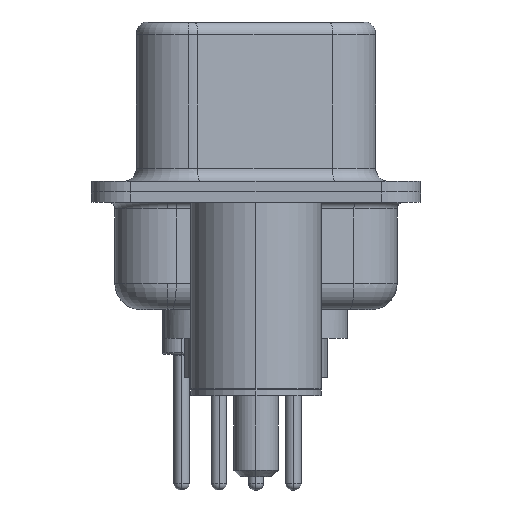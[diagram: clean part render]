
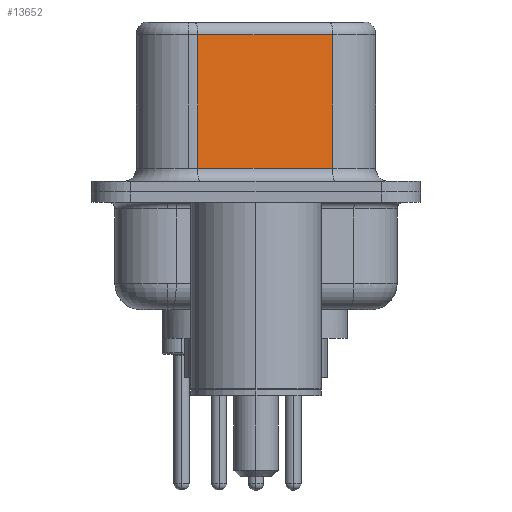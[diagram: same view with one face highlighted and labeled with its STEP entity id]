
A CAD part, left-side view. The second image highlights one B-rep face of the part: STEP entity #13652.
In plain terms, the highlighted planar face has unit normal (-0.985, -0.174, 0).
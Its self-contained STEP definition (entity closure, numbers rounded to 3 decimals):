
#47 = EDGE_CURVE ( 'NONE', #17568, #5700, #17618, .T. ) ;
#399 = CARTESIAN_POINT ( 'NONE',  ( 4.585, -2.927, 0.9 ) ) ;
#1274 = LINE ( 'NONE', #7657, #2582 ) ;
#1430 = CARTESIAN_POINT ( 'NONE',  ( 3.675, 2.233, 0.9 ) ) ;
#1570 = DIRECTION ( 'NONE',  ( 0., 0., -1. ) ) ;
#2396 = EDGE_LOOP ( 'NONE', ( #7359, #12684, #12762, #6263 ) ) ;
#2582 = VECTOR ( 'NONE', #3065, 1000. ) ;
#2789 = VERTEX_POINT ( 'NONE', #1430 ) ;
#3065 = DIRECTION ( 'NONE',  ( 0., 0., -1. ) ) ;
#3313 = CARTESIAN_POINT ( 'NONE',  ( 4.585, -2.927, 6.02 ) ) ;
#3694 = EDGE_CURVE ( 'NONE', #5700, #2789, #18940, .T. ) ;
#3862 = LINE ( 'NONE', #11351, #12015 ) ;
#4662 = EDGE_CURVE ( 'NONE', #2789, #15742, #3862, .T. ) ;
#5011 = CARTESIAN_POINT ( 'NONE',  ( 3.675, 2.233, 6.02 ) ) ;
#5700 = VERTEX_POINT ( 'NONE', #5011 ) ;
#6230 = CARTESIAN_POINT ( 'NONE',  ( 4.585, -2.927, 6.52 ) ) ;
#6263 = ORIENTED_EDGE ( 'NONE', *, *, #4662, .T. ) ;
#7153 = VECTOR ( 'NONE', #1570, 1000. ) ;
#7359 = ORIENTED_EDGE ( 'NONE', *, *, #16768, .F. ) ;
#7657 = CARTESIAN_POINT ( 'NONE',  ( 4.585, -2.927, 6.52 ) ) ;
#7846 = DIRECTION ( 'NONE',  ( 0.985, 0.174, 0. ) ) ;
#11351 = CARTESIAN_POINT ( 'NONE',  ( 4.585, -2.927, 0.9 ) ) ;
#12015 = VECTOR ( 'NONE', #16182, 1000. ) ;
#12684 = ORIENTED_EDGE ( 'NONE', *, *, #47, .T. ) ;
#12762 = ORIENTED_EDGE ( 'NONE', *, *, #3694, .T. ) ;
#13543 = VECTOR ( 'NONE', #14681, 1000. ) ;
#13652 = ADVANCED_FACE ( 'NONE', ( #18604 ), #14410, .F. ) ;
#14410 = PLANE ( 'NONE',  #15688 ) ;
#14681 = DIRECTION ( 'NONE',  ( -0.174, 0.985, 0. ) ) ;
#15688 = AXIS2_PLACEMENT_3D ( 'NONE', #6230, #7846, #15972 ) ;
#15742 = VERTEX_POINT ( 'NONE', #399 ) ;
#15972 = DIRECTION ( 'NONE',  ( -0.174, 0.985, 0. ) ) ;
#16045 = CARTESIAN_POINT ( 'NONE',  ( 4.585, -2.927, 6.02 ) ) ;
#16182 = DIRECTION ( 'NONE',  ( 0.174, -0.985, 0. ) ) ;
#16768 = EDGE_CURVE ( 'NONE', #17568, #15742, #1274, .T. ) ;
#17568 = VERTEX_POINT ( 'NONE', #3313 ) ;
#17618 = LINE ( 'NONE', #16045, #13543 ) ;
#18604 = FACE_OUTER_BOUND ( 'NONE', #2396, .T. ) ;
#18940 = LINE ( 'NONE', #21032, #7153 ) ;
#21032 = CARTESIAN_POINT ( 'NONE',  ( 3.675, 2.233, 6.52 ) ) ;
